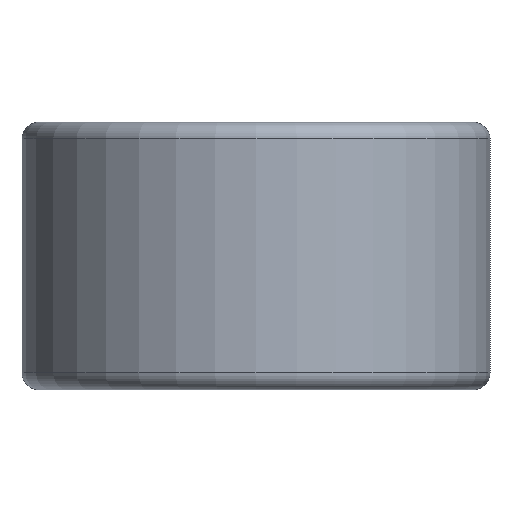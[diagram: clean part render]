
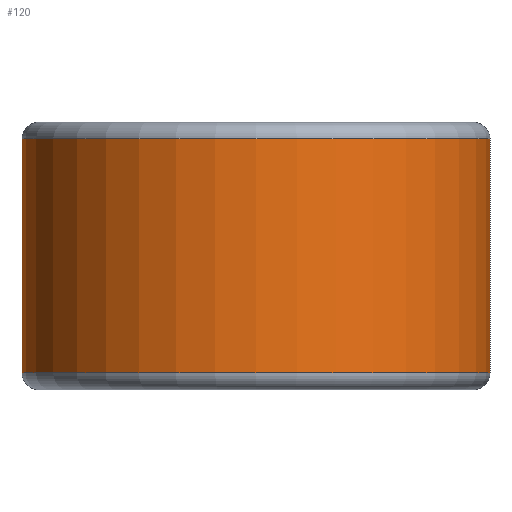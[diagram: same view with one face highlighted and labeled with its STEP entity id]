
A CAD part, front view. The second image highlights one B-rep face of the part: STEP entity #120.
In plain terms, the highlighted cylindrical face has radius 3.5 mm (diameter 7 mm), a full revolution.
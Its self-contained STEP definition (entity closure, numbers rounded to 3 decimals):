
#19=LINE('',#222,#21);
#21=VECTOR('',#177,4.5);
#23=CYLINDRICAL_SURFACE('',#146,3.5);
#26=FACE_OUTER_BOUND('',#34,.T.);
#34=EDGE_LOOP('',(#88,#89,#90,#91,#92));
#43=CIRCLE('',#142,3.5);
#46=CIRCLE('',#145,3.5);
#47=CIRCLE('',#147,3.5);
#57=VERTEX_POINT('',#213);
#58=VERTEX_POINT('',#214);
#60=VERTEX_POINT('',#221);
#67=EDGE_CURVE('',#57,#58,#43,.T.);
#70=EDGE_CURVE('',#58,#57,#46,.T.);
#71=EDGE_CURVE('',#57,#60,#19,.T.);
#72=EDGE_CURVE('',#60,#60,#47,.T.);
#88=ORIENTED_EDGE('',*,*,#67,.F.);
#89=ORIENTED_EDGE('',*,*,#71,.T.);
#90=ORIENTED_EDGE('',*,*,#72,.F.);
#91=ORIENTED_EDGE('',*,*,#71,.F.);
#92=ORIENTED_EDGE('',*,*,#70,.F.);
#120=ADVANCED_FACE('',(#26),#23,.T.);
#142=AXIS2_PLACEMENT_3D('',#215,#167,#168);
#145=AXIS2_PLACEMENT_3D('',#219,#173,#174);
#146=AXIS2_PLACEMENT_3D('',#220,#175,#176);
#147=AXIS2_PLACEMENT_3D('',#223,#178,#179);
#167=DIRECTION('center_axis',(0.,0.,1.));
#168=DIRECTION('ref_axis',(1.,0.,0.));
#173=DIRECTION('center_axis',(0.,0.,1.));
#174=DIRECTION('ref_axis',(1.,0.,0.));
#175=DIRECTION('center_axis',(0.,0.,1.));
#176=DIRECTION('ref_axis',(1.,0.,0.));
#177=DIRECTION('',(0.,0.,-1.));
#178=DIRECTION('center_axis',(0.,0.,-1.));
#179=DIRECTION('ref_axis',(1.,0.,0.));
#213=CARTESIAN_POINT('',(6.5,20.,3.75));
#214=CARTESIAN_POINT('',(13.5,20.,3.75));
#215=CARTESIAN_POINT('Origin',(10.,20.,3.75));
#219=CARTESIAN_POINT('Origin',(10.,20.,3.75));
#220=CARTESIAN_POINT('Origin',(10.,20.,0.));
#221=CARTESIAN_POINT('',(6.5,20.,0.25));
#222=CARTESIAN_POINT('',(6.5,20.,0.));
#223=CARTESIAN_POINT('Origin',(10.,20.,0.25));
